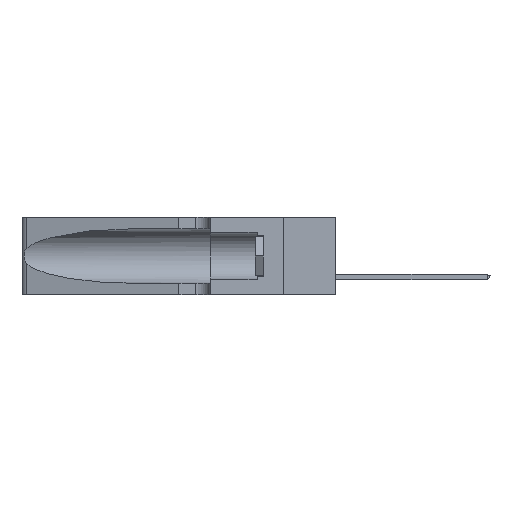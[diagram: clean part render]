
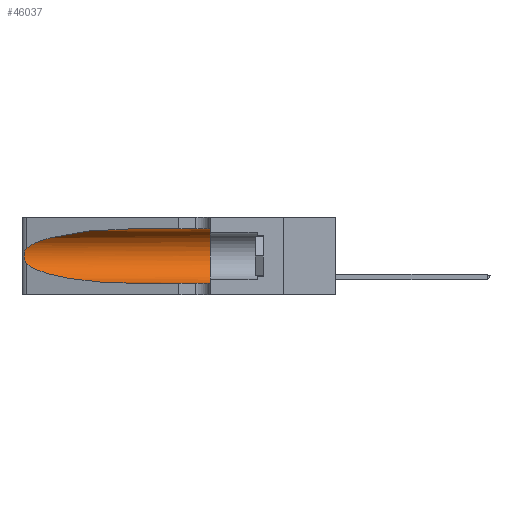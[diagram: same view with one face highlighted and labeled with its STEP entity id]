
A CAD part, left-side view. The second image highlights one B-rep face of the part: STEP entity #46037.
In plain terms, the highlighted cylindrical face has radius 3.308 mm (diameter 6.617 mm), a partial arc.
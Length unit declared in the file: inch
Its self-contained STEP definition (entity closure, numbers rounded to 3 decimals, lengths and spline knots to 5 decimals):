
#308 = AXIS2_PLACEMENT_3D ( 'NONE', #7124, #14844, #33068 ) ;
#1217 = CARTESIAN_POINT ( 'NONE',  ( 0.25555, 1.22994, 0.2215 ) ) ;
#1457 = CYLINDRICAL_SURFACE ( 'NONE', #28528, 0.13025 ) ;
#1539 = CARTESIAN_POINT ( 'NONE',  ( 0.26075, 1.23896, 0.178 ) ) ;
#1904 = EDGE_CURVE ( 'NONE', #17355, #27322, #13204, .T. ) ;
#2466 = DIRECTION ( 'NONE',  ( 0., 0., -1. ) ) ;
#3376 = CARTESIAN_POINT ( 'NONE',  ( 0.25487, 1.22718, 0.14631 ) ) ;
#4745 = CARTESIAN_POINT ( 'NONE',  ( 0.1305, 0.72297, 0.05475 ) ) ;
#5107 = CARTESIAN_POINT ( 'NONE',  ( 0.26017, 1.23833, 0.17102 ) ) ;
#5741 = CARTESIAN_POINT ( 'NONE',  ( 0.25787, 1.23484, 0.2124 ) ) ;
#5881 = EDGE_CURVE ( 'NONE', #6703, #25394, #11996, .T. ) ;
#6475 = CARTESIAN_POINT ( 'NONE',  ( 0.1305, 0.72297, 0.05475 ) ) ;
#6703 = VERTEX_POINT ( 'NONE', #9542 ) ;
#7124 = CARTESIAN_POINT ( 'NONE',  ( 0.1305, 0.35, 0.185 ) ) ;
#7205 = FACE_OUTER_BOUND ( 'NONE', #25257, .T. ) ;
#7232 = CARTESIAN_POINT ( 'NONE',  ( 0.2373, 1.15595, 0.08982 ) ) ;
#8338 = CARTESIAN_POINT ( 'NONE',  ( 0.25487, 1.22718, 0.22369 ) ) ;
#8811 = CARTESIAN_POINT ( 'NONE',  ( 0.26075, 1.23896, 0.19203 ) ) ;
#9542 = CARTESIAN_POINT ( 'NONE',  ( 0.25487, 1.22718, 0.14631 ) ) ;
#9758 = DIRECTION ( 'NONE',  ( 0., -1., 0. ) ) ;
#11385 =( BOUNDED_CURVE ( )  B_SPLINE_CURVE ( 3, ( #27040, #34091, #30479, #26880 ),
 .UNSPECIFIED., .F., .F. ) 
 B_SPLINE_CURVE_WITH_KNOTS ( ( 4, 4 ),
 ( 1.5708, 2.84003 ),
 .UNSPECIFIED. ) 
 CURVE ( )  GEOMETRIC_REPRESENTATION_ITEM ( )  RATIONAL_B_SPLINE_CURVE ( ( 1., 0.87, 0.87, 1. ) ) 
 REPRESENTATION_ITEM ( '' )  );
#11930 = CARTESIAN_POINT ( 'NONE',  ( 0.1305, 0.35, 0.31525 ) ) ;
#11996 =( BOUNDED_CURVE ( )  B_SPLINE_CURVE ( 3, ( #3376, #7232, #40791, #4745 ),
 .UNSPECIFIED., .F., .F. ) 
 B_SPLINE_CURVE_WITH_KNOTS ( ( 4, 4 ),
 ( 3.44316, 4.71239 ),
 .UNSPECIFIED. ) 
 CURVE ( )  GEOMETRIC_REPRESENTATION_ITEM ( )  RATIONAL_B_SPLINE_CURVE ( ( 1., 0.87, 0.87, 1. ) ) 
 REPRESENTATION_ITEM ( '' )  );
#12939 = VERTEX_POINT ( 'NONE', #32763 ) ;
#13204 = LINE ( 'NONE', #39417, #27151 ) ;
#14844 = DIRECTION ( 'NONE',  ( 0., 1., 0. ) ) ;
#15205 = ORIENTED_EDGE ( 'NONE', *, *, #28919, .T. ) ;
#16062 = CARTESIAN_POINT ( 'NONE',  ( 0.25487, 1.22718, 0.14631 ) ) ;
#16514 = VECTOR ( 'NONE', #43002, 39.37008 ) ;
#17007 = CARTESIAN_POINT ( 'NONE',  ( 0.1305, 1.61858, 0.05475 ) ) ;
#17355 = VERTEX_POINT ( 'NONE', #31311 ) ;
#20220 = CARTESIAN_POINT ( 'NONE',  ( 0.25639, 1.23184, 0.21858 ) ) ;
#21023 = ORIENTED_EDGE ( 'NONE', *, *, #5881, .T. ) ;
#23184 = CARTESIAN_POINT ( 'NONE',  ( 0.25487, 1.22718, 0.22369 ) ) ;
#23335 = VERTEX_POINT ( 'NONE', #23184 ) ;
#23808 = CARTESIAN_POINT ( 'NONE',  ( 0.25555, 1.22993, 0.14849 ) ) ;
#25257 = EDGE_LOOP ( 'NONE', ( #35317, #34722, #21023, #15205, #47725, #30906 ) ) ;
#25394 = VERTEX_POINT ( 'NONE', #6475 ) ;
#26880 = CARTESIAN_POINT ( 'NONE',  ( 0.25487, 1.22718, 0.22369 ) ) ;
#27040 = CARTESIAN_POINT ( 'NONE',  ( 0.1305, 0.72297, 0.31525 ) ) ;
#27151 = VECTOR ( 'NONE', #9758, 39.37008 ) ;
#27322 = VERTEX_POINT ( 'NONE', #11930 ) ;
#27415 = CARTESIAN_POINT ( 'NONE',  ( 0.25789, 1.23486, 0.15765 ) ) ;
#28528 = AXIS2_PLACEMENT_3D ( 'NONE', #46188, #31784, #2466 ) ;
#28919 = EDGE_CURVE ( 'NONE', #25394, #12939, #36869, .T. ) ;
#30337 = EDGE_CURVE ( 'NONE', #23335, #6703, #47339, .T. ) ;
#30479 = CARTESIAN_POINT ( 'NONE',  ( 0.2373, 1.15595, 0.28018 ) ) ;
#30906 = ORIENTED_EDGE ( 'NONE', *, *, #1904, .F. ) ;
#31311 = CARTESIAN_POINT ( 'NONE',  ( 0.1305, 0.72297, 0.31525 ) ) ;
#31784 = DIRECTION ( 'NONE',  ( 0., -1., 0. ) ) ;
#32763 = CARTESIAN_POINT ( 'NONE',  ( 0.1305, 0.35, 0.05475 ) ) ;
#33068 = DIRECTION ( 'NONE',  ( 0., 0., 1. ) ) ;
#34091 = CARTESIAN_POINT ( 'NONE',  ( 0.18966, 0.96281, 0.31525 ) ) ;
#34722 = ORIENTED_EDGE ( 'NONE', *, *, #30337, .T. ) ;
#35237 = CARTESIAN_POINT ( 'NONE',  ( 0.26018, 1.23835, 0.19895 ) ) ;
#35317 = ORIENTED_EDGE ( 'NONE', *, *, #42794, .T. ) ;
#36802 = CIRCLE ( 'NONE', #308, 0.13025 ) ;
#36869 = LINE ( 'NONE', #17007, #16514 ) ;
#38310 = CARTESIAN_POINT ( 'NONE',  ( 0.25639, 1.23186, 0.15144 ) ) ;
#39417 = CARTESIAN_POINT ( 'NONE',  ( 0.1305, 1.61858, 0.31525 ) ) ;
#40791 = CARTESIAN_POINT ( 'NONE',  ( 0.18966, 0.96281, 0.05475 ) ) ;
#42048 = CARTESIAN_POINT ( 'NONE',  ( 0.25856, 1.23593, 0.16098 ) ) ;
#42794 = EDGE_CURVE ( 'NONE', #17355, #23335, #11385, .T. ) ;
#43002 = DIRECTION ( 'NONE',  ( 0., -1., 0. ) ) ;
#46037 = ADVANCED_FACE ( 'NONE', ( #7205 ), #1457, .F. ) ;
#46066 = CARTESIAN_POINT ( 'NONE',  ( 0.25854, 1.2359, 0.20912 ) ) ;
#46188 = CARTESIAN_POINT ( 'NONE',  ( 0.1305, 1.61858, 0.185 ) ) ;
#46234 = EDGE_CURVE ( 'NONE', #27322, #12939, #36802, .T. ) ;
#47339 = B_SPLINE_CURVE_WITH_KNOTS ( 'NONE', 3,
 ( #8338, #1217, #20220, #5741, #46066, #35237, #8811, #1539, #5107, #42048, #27415, #38310, #23808, #16062 ),
 .UNSPECIFIED., .F., .F.,
 ( 4, 2, 2, 2, 2, 2, 4 ),
 ( 0., 0.00027, 0.00053, 0.00107, 0.0016, 0.00187, 0.00214 ),
 .UNSPECIFIED. ) ;
#47725 = ORIENTED_EDGE ( 'NONE', *, *, #46234, .F. ) ;
